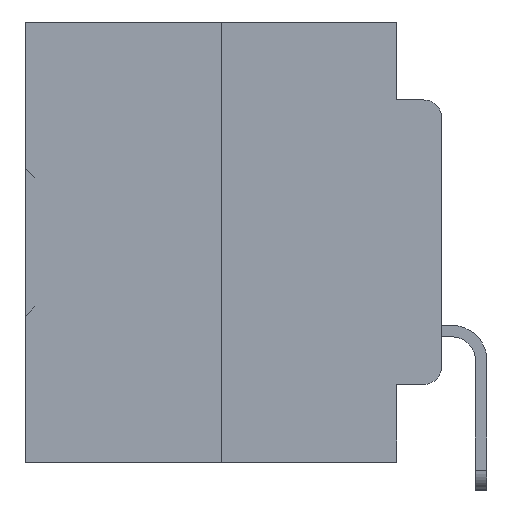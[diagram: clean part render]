
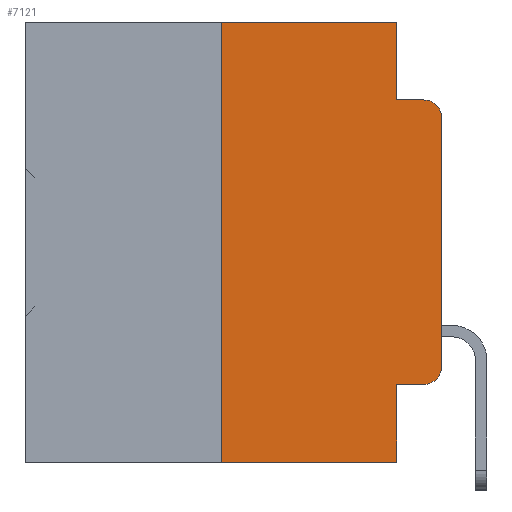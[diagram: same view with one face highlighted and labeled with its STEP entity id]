
A CAD part, left-side view. The second image highlights one B-rep face of the part: STEP entity #7121.
In plain terms, the highlighted planar face has unit normal (-1, 0, 0).
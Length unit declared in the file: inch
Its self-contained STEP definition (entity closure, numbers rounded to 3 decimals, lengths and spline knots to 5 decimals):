
#519 = CARTESIAN_POINT ( 'NONE',  ( 0., 0.051, -0.0885 ) ) ;
#583 = CARTESIAN_POINT ( 'NONE',  ( 0., 0.051, -0.5 ) ) ;
#1281 = DIRECTION ( 'NONE',  ( 0., -1., 0. ) ) ;
#1314 = DIRECTION ( 'NONE',  ( 0., 0., -1. ) ) ;
#1453 = DIRECTION ( 'NONE',  ( 0., 0., -1. ) ) ;
#1673 = CIRCLE ( 'NONE', #2249, 0.02 ) ;
#1727 = VECTOR ( 'NONE', #29646, 39.37008 ) ;
#2249 = AXIS2_PLACEMENT_3D ( 'NONE', #3486, #24369, #6614 ) ;
#3486 = CARTESIAN_POINT ( 'NONE',  ( 0., 0.02, -0.1085 ) ) ;
#3645 = DIRECTION ( 'NONE',  ( 0., -1., 0. ) ) ;
#4014 = VERTEX_POINT ( 'NONE', #7704 ) ;
#4366 = ORIENTED_EDGE ( 'NONE', *, *, #33892, .T. ) ;
#4621 = DIRECTION ( 'NONE',  ( 0., 0., 1. ) ) ;
#4933 = VECTOR ( 'NONE', #9031, 39.37008 ) ;
#5266 = CARTESIAN_POINT ( 'NONE',  ( 0., 0.473, -0.5 ) ) ;
#5584 = VERTEX_POINT ( 'NONE', #583 ) ;
#6542 = VECTOR ( 'NONE', #1453, 39.37008 ) ;
#6614 = DIRECTION ( 'NONE',  ( 0., 0., -1. ) ) ;
#7121 = ADVANCED_FACE ( 'NONE', ( #29711 ), #33400, .F. ) ;
#7520 = LINE ( 'NONE', #30837, #6542 ) ;
#7704 = CARTESIAN_POINT ( 'NONE',  ( 0., 0.25, 0. ) ) ;
#8006 = CARTESIAN_POINT ( 'NONE',  ( 0., 0.02, -0.4115 ) ) ;
#8381 = DIRECTION ( 'NONE',  ( 0., -1., 0. ) ) ;
#8827 = EDGE_CURVE ( 'NONE', #21818, #27653, #10553, .T. ) ;
#8966 = ORIENTED_EDGE ( 'NONE', *, *, #25409, .T. ) ;
#9031 = DIRECTION ( 'NONE',  ( 0., 0., -1. ) ) ;
#9474 = ORIENTED_EDGE ( 'NONE', *, *, #15897, .F. ) ;
#9574 = VECTOR ( 'NONE', #1281, 39.37008 ) ;
#9827 = LINE ( 'NONE', #5266, #24550 ) ;
#9952 = LINE ( 'NONE', #26830, #1727 ) ;
#10553 = LINE ( 'NONE', #35993, #9574 ) ;
#11504 = CARTESIAN_POINT ( 'NONE',  ( 0., 0.473, 0. ) ) ;
#11848 = VECTOR ( 'NONE', #3645, 39.37008 ) ;
#11916 = LINE ( 'NONE', #11504, #26502 ) ;
#13590 = AXIS2_PLACEMENT_3D ( 'NONE', #16601, #19496, #1314 ) ;
#14614 = ORIENTED_EDGE ( 'NONE', *, *, #16240, .F. ) ;
#14690 = VERTEX_POINT ( 'NONE', #14962 ) ;
#14692 = ORIENTED_EDGE ( 'NONE', *, *, #18739, .F. ) ;
#14935 = VERTEX_POINT ( 'NONE', #21900 ) ;
#14962 = CARTESIAN_POINT ( 'NONE',  ( 0., 0.051, 0. ) ) ;
#15363 = DIRECTION ( 'NONE',  ( -1., 0., 0. ) ) ;
#15523 = ORIENTED_EDGE ( 'NONE', *, *, #35569, .F. ) ;
#15897 = EDGE_CURVE ( 'NONE', #20096, #23692, #34528, .T. ) ;
#15948 = ORIENTED_EDGE ( 'NONE', *, *, #28924, .T. ) ;
#16136 = CARTESIAN_POINT ( 'NONE',  ( 0., 0.051, -0.4115 ) ) ;
#16240 = EDGE_CURVE ( 'NONE', #14690, #20096, #20017, .T. ) ;
#16601 = CARTESIAN_POINT ( 'NONE',  ( 0., 0.473, 0. ) ) ;
#18604 = ORIENTED_EDGE ( 'NONE', *, *, #37090, .F. ) ;
#18739 = EDGE_CURVE ( 'NONE', #4014, #14690, #11916, .T. ) ;
#18751 = ORIENTED_EDGE ( 'NONE', *, *, #8827, .T. ) ;
#18877 = LINE ( 'NONE', #33551, #32900 ) ;
#18939 = ORIENTED_EDGE ( 'NONE', *, *, #21660, .T. ) ;
#19496 = DIRECTION ( 'NONE',  ( 1., 0., 0. ) ) ;
#19926 = VERTEX_POINT ( 'NONE', #27674 ) ;
#20017 = LINE ( 'NONE', #23765, #4933 ) ;
#20096 = VERTEX_POINT ( 'NONE', #22805 ) ;
#21475 = EDGE_LOOP ( 'NONE', ( #8966, #4366, #9474, #14614, #14692, #15523, #15948, #18604, #18751, #18939 ) ) ;
#21660 = EDGE_CURVE ( 'NONE', #27653, #19926, #23877, .T. ) ;
#21818 = VERTEX_POINT ( 'NONE', #16136 ) ;
#21900 = CARTESIAN_POINT ( 'NONE',  ( 0., 0., -0.1085 ) ) ;
#22805 = CARTESIAN_POINT ( 'NONE',  ( 0., 0.051, -0.0885 ) ) ;
#23692 = VERTEX_POINT ( 'NONE', #25982 ) ;
#23765 = CARTESIAN_POINT ( 'NONE',  ( 0., 0.051, 0. ) ) ;
#23877 = CIRCLE ( 'NONE', #33959, 0.02 ) ;
#24369 = DIRECTION ( 'NONE',  ( -1., 0., 0. ) ) ;
#24550 = VECTOR ( 'NONE', #8381, 39.37008 ) ;
#25409 = EDGE_CURVE ( 'NONE', #19926, #14935, #9952, .T. ) ;
#25982 = CARTESIAN_POINT ( 'NONE',  ( 0., 0.02, -0.0885 ) ) ;
#26055 = DIRECTION ( 'NONE',  ( 0., -1., 0. ) ) ;
#26502 = VECTOR ( 'NONE', #26055, 39.37008 ) ;
#26830 = CARTESIAN_POINT ( 'NONE',  ( 0., 0., 0. ) ) ;
#27653 = VERTEX_POINT ( 'NONE', #8006 ) ;
#27674 = CARTESIAN_POINT ( 'NONE',  ( 0., 0., -0.3915 ) ) ;
#28924 = EDGE_CURVE ( 'NONE', #34826, #5584, #9827, .T. ) ;
#29646 = DIRECTION ( 'NONE',  ( 0., 0., 1. ) ) ;
#29711 = FACE_OUTER_BOUND ( 'NONE', #21475, .T. ) ;
#30837 = CARTESIAN_POINT ( 'NONE',  ( 0., 0.051, 0. ) ) ;
#32318 = CARTESIAN_POINT ( 'NONE',  ( 0., 0.02, -0.3915 ) ) ;
#32900 = VECTOR ( 'NONE', #4621, 39.37008 ) ;
#33400 = PLANE ( 'NONE',  #13590 ) ;
#33551 = CARTESIAN_POINT ( 'NONE',  ( 0., 0.25, 0. ) ) ;
#33834 = CARTESIAN_POINT ( 'NONE',  ( 0., 0.25, -0.5 ) ) ;
#33892 = EDGE_CURVE ( 'NONE', #14935, #23692, #1673, .T. ) ;
#33959 = AXIS2_PLACEMENT_3D ( 'NONE', #32318, #15363, #34967 ) ;
#34528 = LINE ( 'NONE', #519, #11848 ) ;
#34826 = VERTEX_POINT ( 'NONE', #33834 ) ;
#34967 = DIRECTION ( 'NONE',  ( 0., 0., -1. ) ) ;
#35569 = EDGE_CURVE ( 'NONE', #34826, #4014, #18877, .T. ) ;
#35993 = CARTESIAN_POINT ( 'NONE',  ( 0., 0.051, -0.4115 ) ) ;
#37090 = EDGE_CURVE ( 'NONE', #21818, #5584, #7520, .T. ) ;
